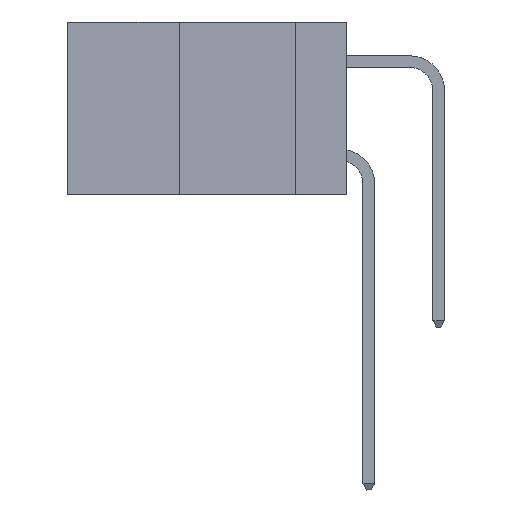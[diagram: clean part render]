
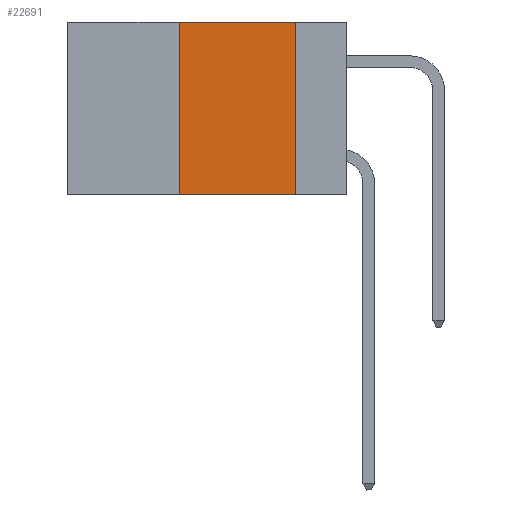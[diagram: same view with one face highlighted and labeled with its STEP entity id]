
A CAD part, left-side view. The second image highlights one B-rep face of the part: STEP entity #22691.
In plain terms, the highlighted planar face has unit normal (-1, 0, 0).
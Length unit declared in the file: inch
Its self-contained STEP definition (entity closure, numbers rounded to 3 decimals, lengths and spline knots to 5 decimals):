
#2803 = VECTOR ( 'NONE', #24846, 39.37008 ) ;
#4236 = ORIENTED_EDGE ( 'NONE', *, *, #28087, .F. ) ;
#4812 = FACE_OUTER_BOUND ( 'NONE', #35850, .T. ) ;
#6225 = VECTOR ( 'NONE', #26829, 39.37008 ) ;
#10735 = AXIS2_PLACEMENT_3D ( 'NONE', #29677, #35601, #32862 ) ;
#12637 = PLANE ( 'NONE',  #10735 ) ;
#12751 = DIRECTION ( 'NONE',  ( 0., -1., 0. ) ) ;
#15789 = LINE ( 'NONE', #18526, #26114 ) ;
#16668 = LINE ( 'NONE', #23714, #6225 ) ;
#18526 = CARTESIAN_POINT ( 'NONE',  ( 0., 0.6, -0.37 ) ) ;
#18625 = CARTESIAN_POINT ( 'NONE',  ( 0., 0.36, 0. ) ) ;
#21290 = EDGE_CURVE ( 'NONE', #23286, #27374, #16668, .T. ) ;
#22655 = VECTOR ( 'NONE', #12751, 39.37008 ) ;
#22691 = ADVANCED_FACE ( 'NONE', ( #4812 ), #12637, .F. ) ;
#23286 = VERTEX_POINT ( 'NONE', #35993 ) ;
#23714 = CARTESIAN_POINT ( 'NONE',  ( 0., 0.36, 0. ) ) ;
#24194 = CARTESIAN_POINT ( 'NONE',  ( 0., 0.11, 0. ) ) ;
#24456 = LINE ( 'NONE', #30680, #2803 ) ;
#24485 = CARTESIAN_POINT ( 'NONE',  ( 0., 0.6, 0. ) ) ;
#24846 = DIRECTION ( 'NONE',  ( 0., 0., -1. ) ) ;
#25867 = ORIENTED_EDGE ( 'NONE', *, *, #28240, .F. ) ;
#26114 = VECTOR ( 'NONE', #29873, 39.37008 ) ;
#26829 = DIRECTION ( 'NONE',  ( 0., 0., 1. ) ) ;
#27365 = VERTEX_POINT ( 'NONE', #30088 ) ;
#27374 = VERTEX_POINT ( 'NONE', #18625 ) ;
#28087 = EDGE_CURVE ( 'NONE', #27374, #35138, #35264, .T. ) ;
#28240 = EDGE_CURVE ( 'NONE', #35138, #27365, #24456, .T. ) ;
#29416 = EDGE_CURVE ( 'NONE', #23286, #27365, #15789, .T. ) ;
#29677 = CARTESIAN_POINT ( 'NONE',  ( 0., 0.6, 0. ) ) ;
#29873 = DIRECTION ( 'NONE',  ( 0., -1., 0. ) ) ;
#30088 = CARTESIAN_POINT ( 'NONE',  ( 0., 0.11, -0.37 ) ) ;
#30680 = CARTESIAN_POINT ( 'NONE',  ( 0., 0.11, 0. ) ) ;
#32063 = ORIENTED_EDGE ( 'NONE', *, *, #21290, .F. ) ;
#32182 = ORIENTED_EDGE ( 'NONE', *, *, #29416, .T. ) ;
#32862 = DIRECTION ( 'NONE',  ( 0., 0., -1. ) ) ;
#35138 = VERTEX_POINT ( 'NONE', #24194 ) ;
#35264 = LINE ( 'NONE', #24485, #22655 ) ;
#35601 = DIRECTION ( 'NONE',  ( 1., 0., 0. ) ) ;
#35850 = EDGE_LOOP ( 'NONE', ( #25867, #4236, #32063, #32182 ) ) ;
#35993 = CARTESIAN_POINT ( 'NONE',  ( 0., 0.36, -0.37 ) ) ;
